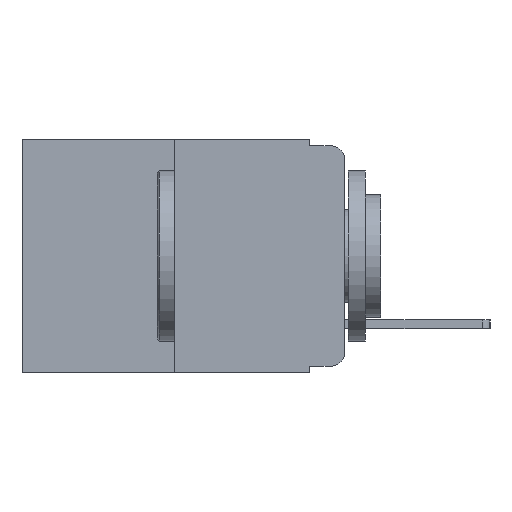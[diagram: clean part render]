
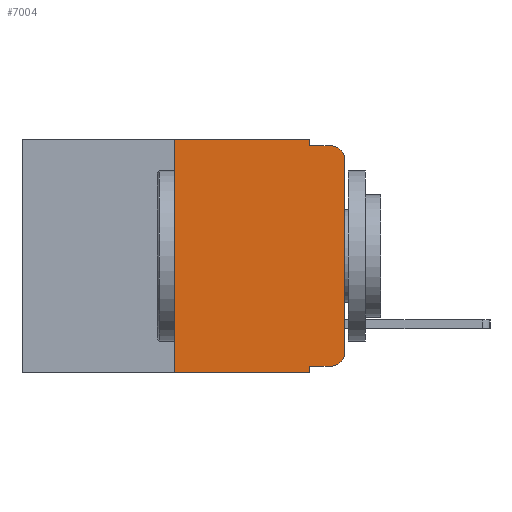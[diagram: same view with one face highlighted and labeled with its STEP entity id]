
A CAD part, left-side view. The second image highlights one B-rep face of the part: STEP entity #7004.
In plain terms, the highlighted planar face has unit normal (-1, 0, 0).
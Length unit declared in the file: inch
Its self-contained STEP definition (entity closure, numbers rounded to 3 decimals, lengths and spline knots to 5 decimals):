
#499 = EDGE_CURVE ( 'NONE', #16425, #6212, #19218, .T. ) ;
#533 = VERTEX_POINT ( 'NONE', #4107 ) ;
#779 = EDGE_LOOP ( 'NONE', ( #8798, #12928, #17343, #7571, #12214, #18478, #8312, #4555, #8819, #17355 ) ) ;
#803 = VECTOR ( 'NONE', #12348, 39.37008 ) ;
#1210 = AXIS2_PLACEMENT_3D ( 'NONE', #14124, #4782, #15642 ) ;
#1398 = PLANE ( 'NONE',  #5530 ) ;
#1632 = CARTESIAN_POINT ( 'NONE',  ( 0., 0.051, -0.01 ) ) ;
#1642 = CARTESIAN_POINT ( 'NONE',  ( 0., 0.02, -0.313 ) ) ;
#3184 = DIRECTION ( 'NONE',  ( -1., 0., 0. ) ) ;
#3326 = CARTESIAN_POINT ( 'NONE',  ( 0., 0.25, -0.343 ) ) ;
#4107 = CARTESIAN_POINT ( 'NONE',  ( 0., 0.02, -0.01 ) ) ;
#4446 = EDGE_CURVE ( 'NONE', #5880, #17855, #5517, .T. ) ;
#4504 = LINE ( 'NONE', #6354, #8267 ) ;
#4555 = ORIENTED_EDGE ( 'NONE', *, *, #8347, .F. ) ;
#4656 = CIRCLE ( 'NONE', #1210, 0.02 ) ;
#4782 = DIRECTION ( 'NONE',  ( -1., 0., 0. ) ) ;
#5159 = DIRECTION ( 'NONE',  ( 0., 0., -1. ) ) ;
#5517 = LINE ( 'NONE', #9755, #803 ) ;
#5530 = AXIS2_PLACEMENT_3D ( 'NONE', #19776, #16857, #12429 ) ;
#5747 = VERTEX_POINT ( 'NONE', #15481 ) ;
#5799 = CARTESIAN_POINT ( 'NONE',  ( 0., 0., -0.313 ) ) ;
#5871 = VECTOR ( 'NONE', #11255, 39.37008 ) ;
#5873 = DIRECTION ( 'NONE',  ( 0., 0., 1. ) ) ;
#5880 = VERTEX_POINT ( 'NONE', #3326 ) ;
#6212 = VERTEX_POINT ( 'NONE', #5799 ) ;
#6245 = EDGE_CURVE ( 'NONE', #5880, #12784, #11263, .T. ) ;
#6354 = CARTESIAN_POINT ( 'NONE',  ( 0., 0.051, 0. ) ) ;
#6435 = DIRECTION ( 'NONE',  ( 0., -1., 0. ) ) ;
#6733 = LINE ( 'NONE', #15225, #18374 ) ;
#6828 = VERTEX_POINT ( 'NONE', #10479 ) ;
#7004 = ADVANCED_FACE ( 'NONE', ( #9513 ), #1398, .F. ) ;
#7571 = ORIENTED_EDGE ( 'NONE', *, *, #18482, .F. ) ;
#7583 = CARTESIAN_POINT ( 'NONE',  ( 0., 0.473, 0. ) ) ;
#7865 = DIRECTION ( 'NONE',  ( 0., 0., -1. ) ) ;
#8267 = VECTOR ( 'NONE', #15508, 39.37008 ) ;
#8312 = ORIENTED_EDGE ( 'NONE', *, *, #4446, .T. ) ;
#8347 = EDGE_CURVE ( 'NONE', #5747, #17855, #17021, .T. ) ;
#8414 = CARTESIAN_POINT ( 'NONE',  ( 0., 0., -0.03 ) ) ;
#8798 = ORIENTED_EDGE ( 'NONE', *, *, #10733, .T. ) ;
#8819 = ORIENTED_EDGE ( 'NONE', *, *, #12527, .T. ) ;
#9219 = LINE ( 'NONE', #18590, #16795 ) ;
#9513 = FACE_OUTER_BOUND ( 'NONE', #779, .T. ) ;
#9755 = CARTESIAN_POINT ( 'NONE',  ( 0., 0.473, -0.343 ) ) ;
#9952 = AXIS2_PLACEMENT_3D ( 'NONE', #1642, #3184, #7865 ) ;
#10479 = CARTESIAN_POINT ( 'NONE',  ( 0., 0.051, 0. ) ) ;
#10733 = EDGE_CURVE ( 'NONE', #6212, #15585, #14122, .T. ) ;
#10761 = VECTOR ( 'NONE', #5873, 39.37008 ) ;
#11255 = DIRECTION ( 'NONE',  ( 0., 0., 1. ) ) ;
#11263 = LINE ( 'NONE', #13632, #10761 ) ;
#11277 = CARTESIAN_POINT ( 'NONE',  ( 0., 0.25, 0. ) ) ;
#11454 = CARTESIAN_POINT ( 'NONE',  ( 0., 0.051, 0. ) ) ;
#12214 = ORIENTED_EDGE ( 'NONE', *, *, #17726, .F. ) ;
#12348 = DIRECTION ( 'NONE',  ( 0., -1., 0. ) ) ;
#12429 = DIRECTION ( 'NONE',  ( 0., 0., -1. ) ) ;
#12527 = EDGE_CURVE ( 'NONE', #5747, #16425, #6733, .T. ) ;
#12652 = CARTESIAN_POINT ( 'NONE',  ( 0., 0., 0. ) ) ;
#12784 = VERTEX_POINT ( 'NONE', #11277 ) ;
#12928 = ORIENTED_EDGE ( 'NONE', *, *, #13786, .T. ) ;
#13061 = VECTOR ( 'NONE', #5159, 39.37008 ) ;
#13632 = CARTESIAN_POINT ( 'NONE',  ( 0., 0.25, 0. ) ) ;
#13712 = DIRECTION ( 'NONE',  ( 0., -1., 0. ) ) ;
#13786 = EDGE_CURVE ( 'NONE', #15585, #533, #4656, .T. ) ;
#14122 = LINE ( 'NONE', #12652, #5871 ) ;
#14124 = CARTESIAN_POINT ( 'NONE',  ( 0., 0.02, -0.03 ) ) ;
#15225 = CARTESIAN_POINT ( 'NONE',  ( 0., 0.051, -0.333 ) ) ;
#15341 = VERTEX_POINT ( 'NONE', #1632 ) ;
#15481 = CARTESIAN_POINT ( 'NONE',  ( 0., 0.051, -0.333 ) ) ;
#15488 = LINE ( 'NONE', #7583, #18468 ) ;
#15508 = DIRECTION ( 'NONE',  ( 0., 0., -1. ) ) ;
#15585 = VERTEX_POINT ( 'NONE', #8414 ) ;
#15625 = CARTESIAN_POINT ( 'NONE',  ( 0., 0.051, -0.343 ) ) ;
#15642 = DIRECTION ( 'NONE',  ( 0., 0., -1. ) ) ;
#15796 = EDGE_CURVE ( 'NONE', #15341, #533, #9219, .T. ) ;
#15821 = CARTESIAN_POINT ( 'NONE',  ( 0., 0.02, -0.333 ) ) ;
#16425 = VERTEX_POINT ( 'NONE', #15821 ) ;
#16795 = VECTOR ( 'NONE', #6435, 39.37008 ) ;
#16857 = DIRECTION ( 'NONE',  ( 1., 0., 0. ) ) ;
#17021 = LINE ( 'NONE', #11454, #13061 ) ;
#17343 = ORIENTED_EDGE ( 'NONE', *, *, #15796, .F. ) ;
#17355 = ORIENTED_EDGE ( 'NONE', *, *, #499, .T. ) ;
#17726 = EDGE_CURVE ( 'NONE', #12784, #6828, #15488, .T. ) ;
#17855 = VERTEX_POINT ( 'NONE', #15625 ) ;
#18374 = VECTOR ( 'NONE', #13712, 39.37008 ) ;
#18468 = VECTOR ( 'NONE', #19648, 39.37008 ) ;
#18478 = ORIENTED_EDGE ( 'NONE', *, *, #6245, .F. ) ;
#18482 = EDGE_CURVE ( 'NONE', #6828, #15341, #4504, .T. ) ;
#18590 = CARTESIAN_POINT ( 'NONE',  ( 0., 0.051, -0.01 ) ) ;
#19218 = CIRCLE ( 'NONE', #9952, 0.02 ) ;
#19648 = DIRECTION ( 'NONE',  ( 0., -1., 0. ) ) ;
#19776 = CARTESIAN_POINT ( 'NONE',  ( 0., 0.473, 0. ) ) ;
